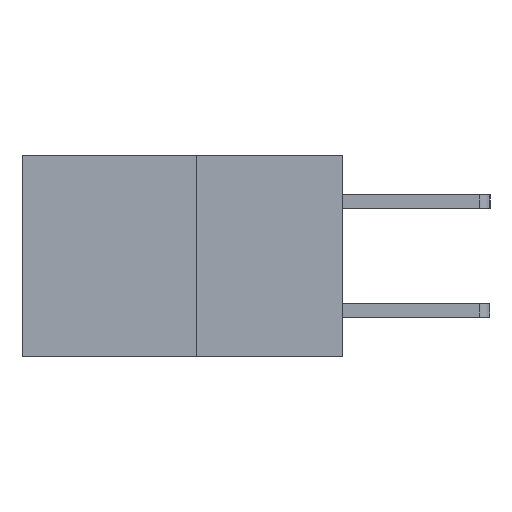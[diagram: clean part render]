
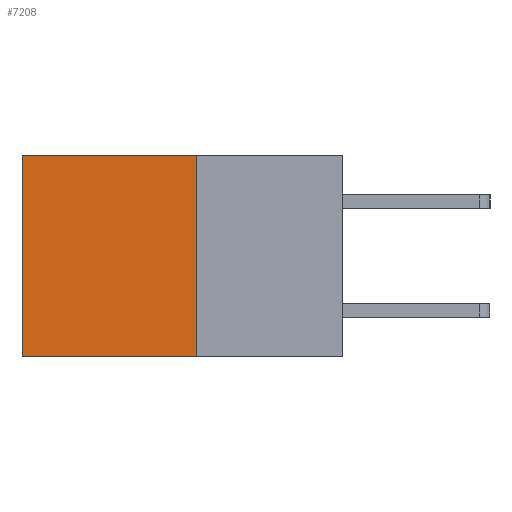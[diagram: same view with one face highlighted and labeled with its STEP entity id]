
A CAD part, left-side view. The second image highlights one B-rep face of the part: STEP entity #7208.
In plain terms, the highlighted planar face has unit normal (-1, 0, 0).
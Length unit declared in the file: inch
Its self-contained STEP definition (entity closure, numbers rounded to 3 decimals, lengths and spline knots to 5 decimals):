
#329 = LINE ( 'NONE', #8166, #7425 ) ;
#688 = LINE ( 'NONE', #1092, #7509 ) ;
#908 = PLANE ( 'NONE',  #5346 ) ;
#940 = DIRECTION ( 'NONE',  ( 0., 1., 0. ) ) ;
#949 = VERTEX_POINT ( 'NONE', #4143 ) ;
#1076 = CARTESIAN_POINT ( 'NONE',  ( 0.277, 0.27, -0.37 ) ) ;
#1092 = CARTESIAN_POINT ( 'NONE',  ( 0.277, 0.27, -0.37 ) ) ;
#1238 = ORIENTED_EDGE ( 'NONE', *, *, #2775, .T. ) ;
#1252 = EDGE_LOOP ( 'NONE', ( #7842, #7003, #1452, #1238 ) ) ;
#1321 = VERTEX_POINT ( 'NONE', #6741 ) ;
#1451 = VECTOR ( 'NONE', #940, 39.37008 ) ;
#1452 = ORIENTED_EDGE ( 'NONE', *, *, #6666, .F. ) ;
#1691 = LINE ( 'NONE', #8101, #6818 ) ;
#1949 = DIRECTION ( 'NONE',  ( 1., 0., 0. ) ) ;
#2190 = DIRECTION ( 'NONE',  ( 0., 0., -1. ) ) ;
#2775 = EDGE_CURVE ( 'NONE', #3790, #949, #1691, .T. ) ;
#3159 = DIRECTION ( 'NONE',  ( 0., 1., 0. ) ) ;
#3359 = EDGE_CURVE ( 'NONE', #1321, #3983, #3416, .T. ) ;
#3416 = LINE ( 'NONE', #7870, #1451 ) ;
#3790 = VERTEX_POINT ( 'NONE', #6395 ) ;
#3983 = VERTEX_POINT ( 'NONE', #4308 ) ;
#4132 = DIRECTION ( 'NONE',  ( 0., 0., -1. ) ) ;
#4143 = CARTESIAN_POINT ( 'NONE',  ( 0.277, 0.59, 0. ) ) ;
#4308 = CARTESIAN_POINT ( 'NONE',  ( 0.277, 0.59, -0.37 ) ) ;
#4396 = FACE_OUTER_BOUND ( 'NONE', #1252, .T. ) ;
#5346 = AXIS2_PLACEMENT_3D ( 'NONE', #1076, #1949, #4132 ) ;
#6395 = CARTESIAN_POINT ( 'NONE',  ( 0.277, 0.27, 0. ) ) ;
#6505 = EDGE_CURVE ( 'NONE', #949, #3983, #329, .T. ) ;
#6666 = EDGE_CURVE ( 'NONE', #3790, #1321, #688, .T. ) ;
#6741 = CARTESIAN_POINT ( 'NONE',  ( 0.277, 0.27, -0.37 ) ) ;
#6818 = VECTOR ( 'NONE', #3159, 39.37008 ) ;
#7003 = ORIENTED_EDGE ( 'NONE', *, *, #3359, .F. ) ;
#7208 = ADVANCED_FACE ( 'NONE', ( #4396 ), #908, .F. ) ;
#7425 = VECTOR ( 'NONE', #7436, 39.37008 ) ;
#7436 = DIRECTION ( 'NONE',  ( 0., 0., -1. ) ) ;
#7509 = VECTOR ( 'NONE', #2190, 39.37008 ) ;
#7842 = ORIENTED_EDGE ( 'NONE', *, *, #6505, .T. ) ;
#7870 = CARTESIAN_POINT ( 'NONE',  ( 0.277, 0.27, -0.37 ) ) ;
#8101 = CARTESIAN_POINT ( 'NONE',  ( 0.277, 0.27, 0. ) ) ;
#8166 = CARTESIAN_POINT ( 'NONE',  ( 0.277, 0.59, -0.37 ) ) ;
